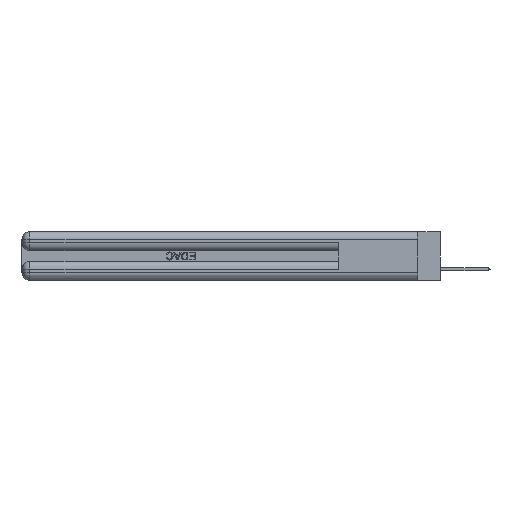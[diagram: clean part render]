
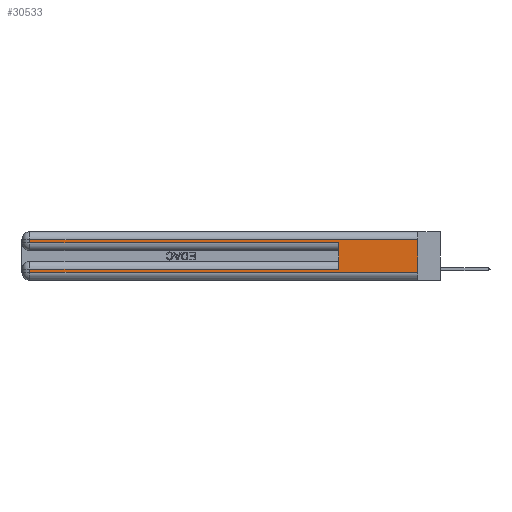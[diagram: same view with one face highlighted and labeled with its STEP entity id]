
A CAD part, left-side view. The second image highlights one B-rep face of the part: STEP entity #30533.
In plain terms, the highlighted planar face has unit normal (-1, 0, 0).
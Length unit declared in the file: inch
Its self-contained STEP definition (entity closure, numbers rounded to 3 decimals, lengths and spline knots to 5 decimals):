
#798 = LINE ( 'NONE', #36360, #33634 ) ;
#1107 = LINE ( 'NONE', #34098, #21242 ) ;
#1125 = VERTEX_POINT ( 'NONE', #12298 ) ;
#1224 = EDGE_CURVE ( 'NONE', #40277, #41732, #7954, .T. ) ;
#2484 = VECTOR ( 'NONE', #27565, 39.37008 ) ;
#3117 = VERTEX_POINT ( 'NONE', #26907 ) ;
#5431 = CARTESIAN_POINT ( 'NONE',  ( 0., 2.94, 0.37 ) ) ;
#6794 = CARTESIAN_POINT ( 'NONE',  ( 0., 0., 0.37 ) ) ;
#7954 = LINE ( 'NONE', #13922, #29354 ) ;
#9028 = EDGE_CURVE ( 'NONE', #3117, #1125, #40078, .T. ) ;
#9731 = DIRECTION ( 'NONE',  ( 0., -1., 0. ) ) ;
#9736 = LINE ( 'NONE', #33875, #21767 ) ;
#10490 = DIRECTION ( 'NONE',  ( 0., 0., -1. ) ) ;
#10745 = VERTEX_POINT ( 'NONE', #49577 ) ;
#10837 = VERTEX_POINT ( 'NONE', #20992 ) ;
#10846 = EDGE_CURVE ( 'NONE', #3117, #41732, #9736, .T. ) ;
#11127 = CARTESIAN_POINT ( 'NONE',  ( 0., 0., 0.06 ) ) ;
#12298 = CARTESIAN_POINT ( 'NONE',  ( 0., 2.94, 0.31 ) ) ;
#12571 = ORIENTED_EDGE ( 'NONE', *, *, #9028, .T. ) ;
#12916 = ORIENTED_EDGE ( 'NONE', *, *, #24271, .F. ) ;
#13922 = CARTESIAN_POINT ( 'NONE',  ( 0., 0., 0.06 ) ) ;
#14067 = VERTEX_POINT ( 'NONE', #29362 ) ;
#14307 = CARTESIAN_POINT ( 'NONE',  ( 0., 0., 0.285 ) ) ;
#15326 = AXIS2_PLACEMENT_3D ( 'NONE', #6794, #20105, #24351 ) ;
#17846 = EDGE_CURVE ( 'NONE', #35912, #10837, #1107, .T. ) ;
#18129 = ORIENTED_EDGE ( 'NONE', *, *, #31564, .T. ) ;
#18189 = EDGE_CURVE ( 'NONE', #10745, #14067, #47244, .T. ) ;
#19147 = EDGE_CURVE ( 'NONE', #1125, #10745, #32155, .T. ) ;
#20105 = DIRECTION ( 'NONE',  ( 1., 0., 0. ) ) ;
#20276 = PLANE ( 'NONE',  #15326 ) ;
#20825 = CARTESIAN_POINT ( 'NONE',  ( 0., 0.6, 0.085 ) ) ;
#20992 = CARTESIAN_POINT ( 'NONE',  ( 0., 2.94, 0.085 ) ) ;
#21242 = VECTOR ( 'NONE', #55051, 39.37008 ) ;
#21767 = VECTOR ( 'NONE', #42459, 39.37008 ) ;
#21983 = VECTOR ( 'NONE', #30794, 39.37008 ) ;
#24271 = EDGE_CURVE ( 'NONE', #35912, #14067, #798, .T. ) ;
#24351 = DIRECTION ( 'NONE',  ( 0., 0., -1. ) ) ;
#25591 = ORIENTED_EDGE ( 'NONE', *, *, #1224, .T. ) ;
#26003 = CARTESIAN_POINT ( 'NONE',  ( 0., 2.94, 0.06 ) ) ;
#26222 = ORIENTED_EDGE ( 'NONE', *, *, #17846, .T. ) ;
#26512 = VECTOR ( 'NONE', #35409, 39.37008 ) ;
#26907 = CARTESIAN_POINT ( 'NONE',  ( 0., 0., 0.31 ) ) ;
#27565 = DIRECTION ( 'NONE',  ( 0., 0., -1. ) ) ;
#29354 = VECTOR ( 'NONE', #9731, 39.37008 ) ;
#29362 = CARTESIAN_POINT ( 'NONE',  ( 0., 0.6, 0.285 ) ) ;
#30533 = ADVANCED_FACE ( 'NONE', ( #31895 ), #20276, .F. ) ;
#30794 = DIRECTION ( 'NONE',  ( 0., 1., 0. ) ) ;
#31174 = CARTESIAN_POINT ( 'NONE',  ( 0., 0., 0.31 ) ) ;
#31356 = CARTESIAN_POINT ( 'NONE',  ( 0., 2.94, 0.37 ) ) ;
#31564 = EDGE_CURVE ( 'NONE', #10837, #40277, #50005, .T. ) ;
#31895 = FACE_OUTER_BOUND ( 'NONE', #53817, .T. ) ;
#32155 = LINE ( 'NONE', #5431, #46226 ) ;
#33634 = VECTOR ( 'NONE', #53738, 39.37008 ) ;
#33875 = CARTESIAN_POINT ( 'NONE',  ( 0., 0., 0.37 ) ) ;
#34098 = CARTESIAN_POINT ( 'NONE',  ( 0., 0., 0.085 ) ) ;
#34223 = ORIENTED_EDGE ( 'NONE', *, *, #10846, .F. ) ;
#35409 = DIRECTION ( 'NONE',  ( 0., -1., 0. ) ) ;
#35912 = VERTEX_POINT ( 'NONE', #20825 ) ;
#36360 = CARTESIAN_POINT ( 'NONE',  ( 0., 0.6, 0.145 ) ) ;
#40078 = LINE ( 'NONE', #31174, #21983 ) ;
#40277 = VERTEX_POINT ( 'NONE', #26003 ) ;
#41732 = VERTEX_POINT ( 'NONE', #11127 ) ;
#42459 = DIRECTION ( 'NONE',  ( 0., 0., -1. ) ) ;
#44437 = ORIENTED_EDGE ( 'NONE', *, *, #18189, .T. ) ;
#45720 = ORIENTED_EDGE ( 'NONE', *, *, #19147, .T. ) ;
#46226 = VECTOR ( 'NONE', #10490, 39.37008 ) ;
#47244 = LINE ( 'NONE', #14307, #26512 ) ;
#49577 = CARTESIAN_POINT ( 'NONE',  ( 0., 2.94, 0.285 ) ) ;
#50005 = LINE ( 'NONE', #31356, #2484 ) ;
#53738 = DIRECTION ( 'NONE',  ( 0., 0., 1. ) ) ;
#53817 = EDGE_LOOP ( 'NONE', ( #34223, #12571, #45720, #44437, #12916, #26222, #18129, #25591 ) ) ;
#55051 = DIRECTION ( 'NONE',  ( 0., 1., 0. ) ) ;
